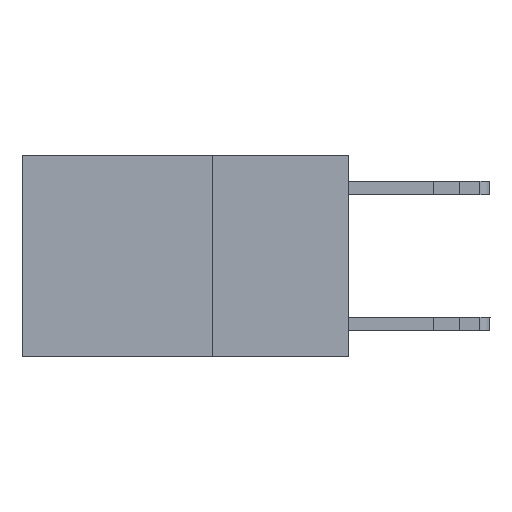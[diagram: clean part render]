
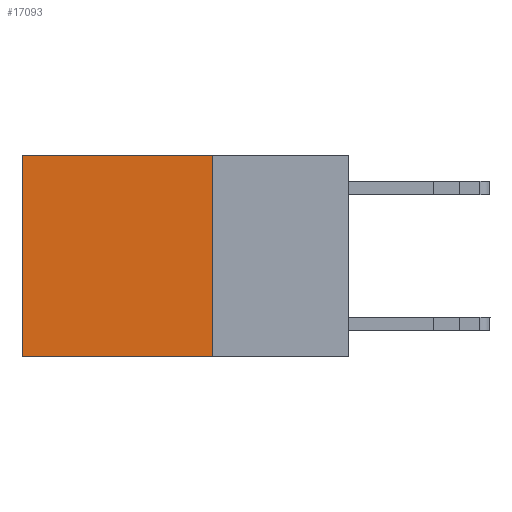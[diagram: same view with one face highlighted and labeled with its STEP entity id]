
A CAD part, left-side view. The second image highlights one B-rep face of the part: STEP entity #17093.
In plain terms, the highlighted planar face has unit normal (-1, 0, 0).
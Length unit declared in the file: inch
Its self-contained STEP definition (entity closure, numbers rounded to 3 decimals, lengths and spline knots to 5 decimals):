
#225 = EDGE_CURVE ( 'NONE', #22344, #22163, #1972, .T. ) ;
#667 = LINE ( 'NONE', #8279, #1593 ) ;
#1593 = VECTOR ( 'NONE', #8253, 39.37008 ) ;
#1886 = VECTOR ( 'NONE', #20580, 39.37008 ) ;
#1972 = LINE ( 'NONE', #19591, #1886 ) ;
#2868 = LINE ( 'NONE', #5942, #2989 ) ;
#2989 = VECTOR ( 'NONE', #6052, 39.37008 ) ;
#3401 = DIRECTION ( 'NONE',  ( 0., 0., -1. ) ) ;
#3723 = CARTESIAN_POINT ( 'NONE',  ( 0.2625, 0.25, 0. ) ) ;
#5942 = CARTESIAN_POINT ( 'NONE',  ( 0.2625, 0.25, 0. ) ) ;
#6052 = DIRECTION ( 'NONE',  ( 0., 1., 0. ) ) ;
#6635 = CARTESIAN_POINT ( 'NONE',  ( 0.2625, 0.25, 0. ) ) ;
#6843 = CARTESIAN_POINT ( 'NONE',  ( 0.2625, 0.6, 0. ) ) ;
#7017 = ORIENTED_EDGE ( 'NONE', *, *, #225, .T. ) ;
#7619 = ORIENTED_EDGE ( 'NONE', *, *, #18151, .T. ) ;
#7721 = EDGE_CURVE ( 'NONE', #14535, #21859, #18215, .T. ) ;
#8080 = EDGE_LOOP ( 'NONE', ( #7017, #12798, #20737, #7619 ) ) ;
#8253 = DIRECTION ( 'NONE',  ( 0., 1., 0. ) ) ;
#8279 = CARTESIAN_POINT ( 'NONE',  ( 0.2625, 0.25, -0.37 ) ) ;
#8756 = CARTESIAN_POINT ( 'NONE',  ( 0.2625, 0.6, -0.37 ) ) ;
#12737 = CARTESIAN_POINT ( 'NONE',  ( 0.2625, 0.25, -0.37 ) ) ;
#12798 = ORIENTED_EDGE ( 'NONE', *, *, #19699, .F. ) ;
#12968 = FACE_OUTER_BOUND ( 'NONE', #8080, .T. ) ;
#14535 = VERTEX_POINT ( 'NONE', #6635 ) ;
#17093 = ADVANCED_FACE ( 'NONE', ( #12968 ), #19500, .F. ) ;
#17544 = AXIS2_PLACEMENT_3D ( 'NONE', #19318, #19315, #19295 ) ;
#18151 = EDGE_CURVE ( 'NONE', #14535, #22344, #2868, .T. ) ;
#18182 = VECTOR ( 'NONE', #3401, 39.37008 ) ;
#18215 = LINE ( 'NONE', #3723, #18182 ) ;
#19295 = DIRECTION ( 'NONE',  ( 0., 0., -1. ) ) ;
#19315 = DIRECTION ( 'NONE',  ( 1., 0., 0. ) ) ;
#19318 = CARTESIAN_POINT ( 'NONE',  ( 0.2625, 0.25, 0. ) ) ;
#19500 = PLANE ( 'NONE',  #17544 ) ;
#19591 = CARTESIAN_POINT ( 'NONE',  ( 0.2625, 0.6, 0. ) ) ;
#19699 = EDGE_CURVE ( 'NONE', #21859, #22163, #667, .T. ) ;
#20580 = DIRECTION ( 'NONE',  ( 0., 0., -1. ) ) ;
#20737 = ORIENTED_EDGE ( 'NONE', *, *, #7721, .F. ) ;
#21859 = VERTEX_POINT ( 'NONE', #12737 ) ;
#22163 = VERTEX_POINT ( 'NONE', #8756 ) ;
#22344 = VERTEX_POINT ( 'NONE', #6843 ) ;
